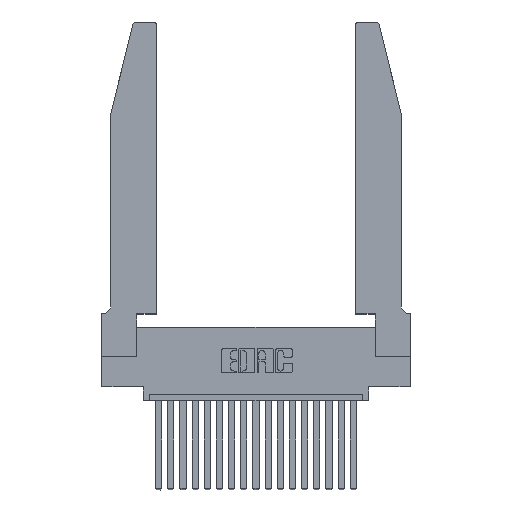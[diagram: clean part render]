
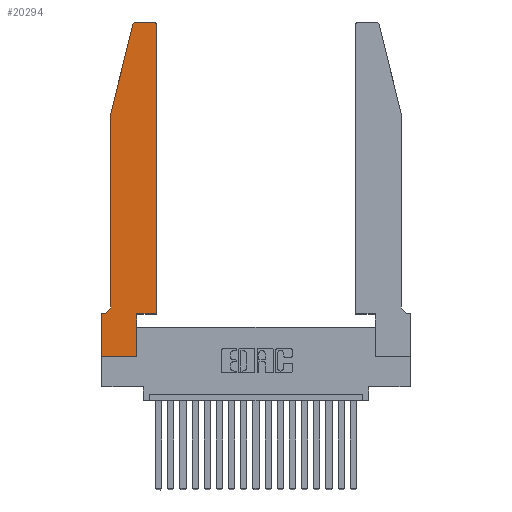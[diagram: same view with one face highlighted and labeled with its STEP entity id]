
A CAD part, top view. The second image highlights one B-rep face of the part: STEP entity #20294.
In plain terms, the highlighted planar face has unit normal (0, 0, 1).
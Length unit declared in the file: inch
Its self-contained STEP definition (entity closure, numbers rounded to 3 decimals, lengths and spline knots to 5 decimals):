
#200 = CARTESIAN_POINT ( 'NONE',  ( 0.2605, 2.75, 0.37 ) ) ;
#491 = DIRECTION ( 'NONE',  ( 0., 0., 1. ) ) ;
#756 = LINE ( 'NONE', #13410, #3799 ) ;
#1154 = ORIENTED_EDGE ( 'NONE', *, *, #11148, .T. ) ;
#1186 = AXIS2_PLACEMENT_3D ( 'NONE', #16095, #12930, #3348 ) ;
#1261 = EDGE_CURVE ( 'NONE', #9259, #9936, #19887, .T. ) ;
#1398 = VERTEX_POINT ( 'NONE', #6472 ) ;
#1650 = ORIENTED_EDGE ( 'NONE', *, *, #15025, .T. ) ;
#1986 = DIRECTION ( 'NONE',  ( -1., 0., 0. ) ) ;
#2148 = CARTESIAN_POINT ( 'NONE',  ( 0.0755, 2., 0.37 ) ) ;
#2374 = CIRCLE ( 'NONE', #1186, 0.07 ) ;
#2641 = EDGE_CURVE ( 'NONE', #18590, #12829, #2800, .T. ) ;
#2772 = VECTOR ( 'NONE', #18288, 39.37008 ) ;
#2800 = LINE ( 'NONE', #200, #10813 ) ;
#3134 = ORIENTED_EDGE ( 'NONE', *, *, #1261, .T. ) ;
#3226 = CARTESIAN_POINT ( 'NONE',  ( 0.2865, 0.35, 0.37 ) ) ;
#3258 = ORIENTED_EDGE ( 'NONE', *, *, #16395, .T. ) ;
#3348 = DIRECTION ( 'NONE',  ( -1., 0., 0. ) ) ;
#3402 = DIRECTION ( 'NONE',  ( 0., -1., 0. ) ) ;
#3437 = ORIENTED_EDGE ( 'NONE', *, *, #5862, .T. ) ;
#3799 = VECTOR ( 'NONE', #16675, 39.37008 ) ;
#3840 = DIRECTION ( 'NONE',  ( 1., 0., 0. ) ) ;
#3927 = LINE ( 'NONE', #9017, #12933 ) ;
#4200 = DIRECTION ( 'NONE',  ( -1., 0., 0. ) ) ;
#4349 = CARTESIAN_POINT ( 'NONE',  ( 0.0755, 0.35, 0.37 ) ) ;
#4367 = EDGE_CURVE ( 'NONE', #9936, #1398, #7973, .T. ) ;
#4531 = VERTEX_POINT ( 'NONE', #18546 ) ;
#4813 = VECTOR ( 'NONE', #4200, 39.37008 ) ;
#5225 = VERTEX_POINT ( 'NONE', #14151 ) ;
#5252 = CARTESIAN_POINT ( 'NONE',  ( 0., 0.35, 0.37 ) ) ;
#5862 = EDGE_CURVE ( 'NONE', #20181, #9259, #2374, .T. ) ;
#5986 = DIRECTION ( 'NONE',  ( 1., 0., 0. ) ) ;
#6472 = CARTESIAN_POINT ( 'NONE',  ( 0., 0., 0.37 ) ) ;
#6586 = CARTESIAN_POINT ( 'NONE',  ( 0.0755, 0.42, 0.37 ) ) ;
#7252 = AXIS2_PLACEMENT_3D ( 'NONE', #14927, #18408, #16571 ) ;
#7312 = ORIENTED_EDGE ( 'NONE', *, *, #15648, .T. ) ;
#7973 = LINE ( 'NONE', #9822, #11703 ) ;
#8701 = ORIENTED_EDGE ( 'NONE', *, *, #15673, .T. ) ;
#8739 = LINE ( 'NONE', #14517, #15012 ) ;
#9017 = CARTESIAN_POINT ( 'NONE',  ( 0.0755, 2., 0.37 ) ) ;
#9259 = VERTEX_POINT ( 'NONE', #18952 ) ;
#9716 = DIRECTION ( 'NONE',  ( 0., 1., 0. ) ) ;
#9771 = ORIENTED_EDGE ( 'NONE', *, *, #16115, .T. ) ;
#9822 = CARTESIAN_POINT ( 'NONE',  ( 0., 0., 0.37 ) ) ;
#9936 = VERTEX_POINT ( 'NONE', #5252 ) ;
#10127 = PLANE ( 'NONE',  #17376 ) ;
#10702 = DIRECTION ( 'NONE',  ( -0.239, -0.971, 0. ) ) ;
#10813 = VECTOR ( 'NONE', #1986, 39.37008 ) ;
#11045 = LINE ( 'NONE', #2148, #2772 ) ;
#11148 = EDGE_CURVE ( 'NONE', #1398, #15739, #756, .T. ) ;
#11472 = VERTEX_POINT ( 'NONE', #17187 ) ;
#11674 = DIRECTION ( 'NONE',  ( 0., 0., 1. ) ) ;
#11703 = VECTOR ( 'NONE', #3402, 39.37008 ) ;
#12135 = VECTOR ( 'NONE', #9716, 39.37008 ) ;
#12394 = CARTESIAN_POINT ( 'NONE',  ( 0.4505, 0.35, 0.37 ) ) ;
#12411 = EDGE_LOOP ( 'NONE', ( #13111, #14985, #9771, #12598, #3437, #3134, #20229, #1154, #7312, #1650, #3258, #8701 ) ) ;
#12598 = ORIENTED_EDGE ( 'NONE', *, *, #20359, .T. ) ;
#12829 = VERTEX_POINT ( 'NONE', #18115 ) ;
#12930 = DIRECTION ( 'NONE',  ( 0., 0., -1. ) ) ;
#12933 = VECTOR ( 'NONE', #10702, 39.37008 ) ;
#13111 = ORIENTED_EDGE ( 'NONE', *, *, #2641, .T. ) ;
#13140 = CIRCLE ( 'NONE', #19705, 0.03 ) ;
#13410 = CARTESIAN_POINT ( 'NONE',  ( 0., 0., 0.37 ) ) ;
#13414 = VECTOR ( 'NONE', #5986, 39.37008 ) ;
#14151 = CARTESIAN_POINT ( 'NONE',  ( 0.4505, 0.35, 0.37 ) ) ;
#14496 = VERTEX_POINT ( 'NONE', #19538 ) ;
#14517 = CARTESIAN_POINT ( 'NONE',  ( 0.4505, 0.35, 0.37 ) ) ;
#14671 = EDGE_CURVE ( 'NONE', #12829, #11472, #19753, .T. ) ;
#14814 = CARTESIAN_POINT ( 'NONE',  ( 0., 0.35, 0.37 ) ) ;
#14927 = CARTESIAN_POINT ( 'NONE',  ( 0.284, 2.72, 0.37 ) ) ;
#14985 = ORIENTED_EDGE ( 'NONE', *, *, #14671, .T. ) ;
#15012 = VECTOR ( 'NONE', #16212, 39.37008 ) ;
#15025 = EDGE_CURVE ( 'NONE', #14496, #5225, #17725, .T. ) ;
#15648 = EDGE_CURVE ( 'NONE', #15739, #14496, #16937, .T. ) ;
#15673 = EDGE_CURVE ( 'NONE', #19312, #18590, #13140, .T. ) ;
#15739 = VERTEX_POINT ( 'NONE', #19852 ) ;
#16095 = CARTESIAN_POINT ( 'NONE',  ( 0.0055, 0.42, 0.37 ) ) ;
#16115 = EDGE_CURVE ( 'NONE', #11472, #4531, #3927, .T. ) ;
#16212 = DIRECTION ( 'NONE',  ( 0., 1., 0. ) ) ;
#16254 = CARTESIAN_POINT ( 'NONE',  ( 0.4205, 2.75, 0.37 ) ) ;
#16395 = EDGE_CURVE ( 'NONE', #5225, #19312, #8739, .T. ) ;
#16571 = DIRECTION ( 'NONE',  ( 1., 0., 0. ) ) ;
#16602 = DIRECTION ( 'NONE',  ( 1., 0., 0. ) ) ;
#16675 = DIRECTION ( 'NONE',  ( 1., 0., 0. ) ) ;
#16937 = LINE ( 'NONE', #3226, #12135 ) ;
#17187 = CARTESIAN_POINT ( 'NONE',  ( 0.25487, 2.72718, 0.37 ) ) ;
#17376 = AXIS2_PLACEMENT_3D ( 'NONE', #14814, #491, #3840 ) ;
#17725 = LINE ( 'NONE', #12394, #13414 ) ;
#17805 = CARTESIAN_POINT ( 'NONE',  ( 0.4505, 2.72, 0.37 ) ) ;
#18115 = CARTESIAN_POINT ( 'NONE',  ( 0.284, 2.75, 0.37 ) ) ;
#18288 = DIRECTION ( 'NONE',  ( 0., -1., 0. ) ) ;
#18408 = DIRECTION ( 'NONE',  ( 0., 0., 1. ) ) ;
#18546 = CARTESIAN_POINT ( 'NONE',  ( 0.0755, 2., 0.37 ) ) ;
#18590 = VERTEX_POINT ( 'NONE', #16254 ) ;
#18952 = CARTESIAN_POINT ( 'NONE',  ( 0.0055, 0.35, 0.37 ) ) ;
#19312 = VERTEX_POINT ( 'NONE', #17805 ) ;
#19538 = CARTESIAN_POINT ( 'NONE',  ( 0.2865, 0.35, 0.37 ) ) ;
#19596 = FACE_OUTER_BOUND ( 'NONE', #12411, .T. ) ;
#19705 = AXIS2_PLACEMENT_3D ( 'NONE', #19781, #11674, #16602 ) ;
#19753 = CIRCLE ( 'NONE', #7252, 0.03 ) ;
#19781 = CARTESIAN_POINT ( 'NONE',  ( 0.4205, 2.72, 0.37 ) ) ;
#19852 = CARTESIAN_POINT ( 'NONE',  ( 0.2865, 0., 0.37 ) ) ;
#19887 = LINE ( 'NONE', #4349, #4813 ) ;
#20181 = VERTEX_POINT ( 'NONE', #6586 ) ;
#20229 = ORIENTED_EDGE ( 'NONE', *, *, #4367, .T. ) ;
#20294 = ADVANCED_FACE ( 'NONE', ( #19596 ), #10127, .T. ) ;
#20359 = EDGE_CURVE ( 'NONE', #4531, #20181, #11045, .T. ) ;
